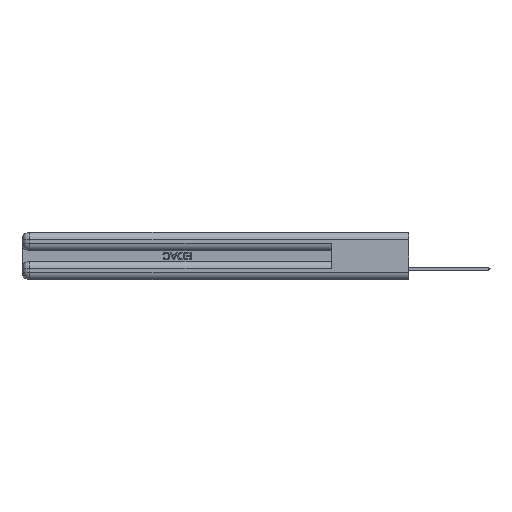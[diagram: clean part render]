
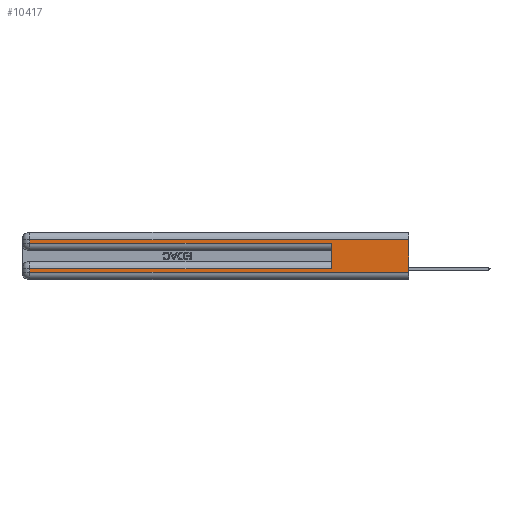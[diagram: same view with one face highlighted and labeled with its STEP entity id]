
A CAD part, left-side view. The second image highlights one B-rep face of the part: STEP entity #10417.
In plain terms, the highlighted planar face has unit normal (-1, 0, 0).
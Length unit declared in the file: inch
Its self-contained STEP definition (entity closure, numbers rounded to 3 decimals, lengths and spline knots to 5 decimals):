
#815 = DIRECTION ( 'NONE',  ( 0., -1., 0. ) ) ;
#1534 = FACE_OUTER_BOUND ( 'NONE', #7772, .T. ) ;
#2658 = DIRECTION ( 'NONE',  ( 0., 1., 0. ) ) ;
#3292 = VECTOR ( 'NONE', #4026, 39.37008 ) ;
#3362 = CARTESIAN_POINT ( 'NONE',  ( 0., 0.6, 0.085 ) ) ;
#3851 = EDGE_CURVE ( 'NONE', #44762, #40553, #27361, .T. ) ;
#4026 = DIRECTION ( 'NONE',  ( 0., 0., -1. ) ) ;
#6464 = DIRECTION ( 'NONE',  ( 0., 1., 0. ) ) ;
#6723 = LINE ( 'NONE', #15487, #35071 ) ;
#6849 = DIRECTION ( 'NONE',  ( 0., 0., -1. ) ) ;
#6895 = VECTOR ( 'NONE', #44211, 39.37008 ) ;
#7772 = EDGE_LOOP ( 'NONE', ( #32049, #32671, #45605, #13317, #12760, #15012, #38212, #11476 ) ) ;
#8489 = EDGE_CURVE ( 'NONE', #39435, #9785, #31175, .T. ) ;
#9450 = VECTOR ( 'NONE', #19419, 39.37008 ) ;
#9643 = DIRECTION ( 'NONE',  ( 0., 0., -1. ) ) ;
#9785 = VERTEX_POINT ( 'NONE', #23268 ) ;
#10139 = CARTESIAN_POINT ( 'NONE',  ( 0., 0., 0.31 ) ) ;
#10323 = EDGE_CURVE ( 'NONE', #14382, #37340, #22927, .T. ) ;
#10367 = AXIS2_PLACEMENT_3D ( 'NONE', #23073, #46564, #9643 ) ;
#10376 = EDGE_CURVE ( 'NONE', #9785, #13538, #6723, .T. ) ;
#10417 = ADVANCED_FACE ( 'NONE', ( #1534 ), #19388, .F. ) ;
#10703 = CARTESIAN_POINT ( 'NONE',  ( 0., 2.94, 0.37 ) ) ;
#10954 = LINE ( 'NONE', #24417, #32898 ) ;
#11476 = ORIENTED_EDGE ( 'NONE', *, *, #24607, .T. ) ;
#12760 = ORIENTED_EDGE ( 'NONE', *, *, #47585, .F. ) ;
#13317 = ORIENTED_EDGE ( 'NONE', *, *, #10376, .T. ) ;
#13538 = VERTEX_POINT ( 'NONE', #18640 ) ;
#14382 = VERTEX_POINT ( 'NONE', #30795 ) ;
#14729 = CARTESIAN_POINT ( 'NONE',  ( 0., 0., 0.06 ) ) ;
#15012 = ORIENTED_EDGE ( 'NONE', *, *, #27172, .T. ) ;
#15227 = DIRECTION ( 'NONE',  ( 0., 0., 1. ) ) ;
#15487 = CARTESIAN_POINT ( 'NONE',  ( 0., 0., 0.285 ) ) ;
#15557 = CARTESIAN_POINT ( 'NONE',  ( 0., 0.6, 0.145 ) ) ;
#17868 = CARTESIAN_POINT ( 'NONE',  ( 0., 2.94, 0.31 ) ) ;
#18640 = CARTESIAN_POINT ( 'NONE',  ( 0., 0.6, 0.285 ) ) ;
#19388 = PLANE ( 'NONE',  #10367 ) ;
#19419 = DIRECTION ( 'NONE',  ( 0., 0., -1. ) ) ;
#20570 = CARTESIAN_POINT ( 'NONE',  ( 0., 0., 0.37 ) ) ;
#21405 = CARTESIAN_POINT ( 'NONE',  ( 0., 0., 0.31 ) ) ;
#21503 = EDGE_CURVE ( 'NONE', #44762, #39435, #30809, .T. ) ;
#22927 = LINE ( 'NONE', #41076, #3292 ) ;
#23073 = CARTESIAN_POINT ( 'NONE',  ( 0., 0., 0.37 ) ) ;
#23268 = CARTESIAN_POINT ( 'NONE',  ( 0., 2.94, 0.285 ) ) ;
#24417 = CARTESIAN_POINT ( 'NONE',  ( 0., 0., 0.085 ) ) ;
#24607 = EDGE_CURVE ( 'NONE', #37340, #40553, #24785, .T. ) ;
#24785 = LINE ( 'NONE', #14729, #6895 ) ;
#25073 = VERTEX_POINT ( 'NONE', #3362 ) ;
#27172 = EDGE_CURVE ( 'NONE', #25073, #14382, #10954, .T. ) ;
#27361 = LINE ( 'NONE', #20570, #9450 ) ;
#27623 = CARTESIAN_POINT ( 'NONE',  ( 0., 2.94, 0.06 ) ) ;
#28169 = LINE ( 'NONE', #15557, #46186 ) ;
#30795 = CARTESIAN_POINT ( 'NONE',  ( 0., 2.94, 0.085 ) ) ;
#30809 = LINE ( 'NONE', #21405, #37263 ) ;
#31175 = LINE ( 'NONE', #10703, #47433 ) ;
#32049 = ORIENTED_EDGE ( 'NONE', *, *, #3851, .F. ) ;
#32671 = ORIENTED_EDGE ( 'NONE', *, *, #21503, .T. ) ;
#32898 = VECTOR ( 'NONE', #6464, 39.37008 ) ;
#35071 = VECTOR ( 'NONE', #815, 39.37008 ) ;
#36896 = CARTESIAN_POINT ( 'NONE',  ( 0., 0., 0.06 ) ) ;
#37263 = VECTOR ( 'NONE', #2658, 39.37008 ) ;
#37340 = VERTEX_POINT ( 'NONE', #27623 ) ;
#38212 = ORIENTED_EDGE ( 'NONE', *, *, #10323, .T. ) ;
#39435 = VERTEX_POINT ( 'NONE', #17868 ) ;
#40553 = VERTEX_POINT ( 'NONE', #36896 ) ;
#41076 = CARTESIAN_POINT ( 'NONE',  ( 0., 2.94, 0.37 ) ) ;
#44211 = DIRECTION ( 'NONE',  ( 0., -1., 0. ) ) ;
#44762 = VERTEX_POINT ( 'NONE', #10139 ) ;
#45605 = ORIENTED_EDGE ( 'NONE', *, *, #8489, .T. ) ;
#46186 = VECTOR ( 'NONE', #15227, 39.37008 ) ;
#46564 = DIRECTION ( 'NONE',  ( 1., 0., 0. ) ) ;
#47433 = VECTOR ( 'NONE', #6849, 39.37008 ) ;
#47585 = EDGE_CURVE ( 'NONE', #25073, #13538, #28169, .T. ) ;
